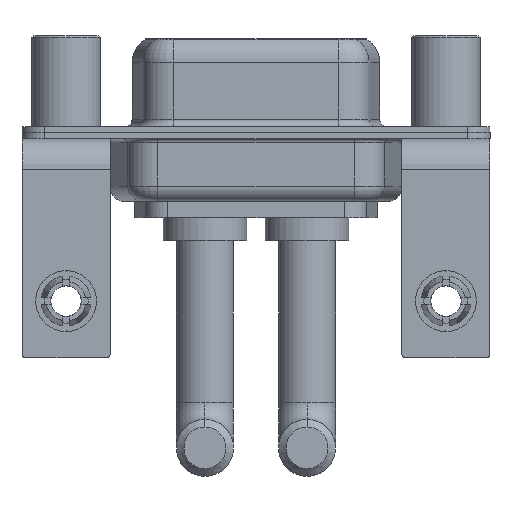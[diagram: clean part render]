
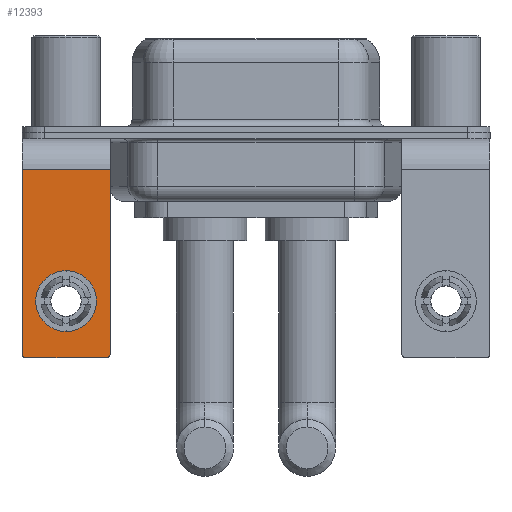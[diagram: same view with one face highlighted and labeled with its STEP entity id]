
A CAD part, front view. The second image highlights one B-rep face of the part: STEP entity #12393.
In plain terms, the highlighted planar face has unit normal (0, -1, 0).
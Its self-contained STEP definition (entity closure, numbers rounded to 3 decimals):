
#445 = CARTESIAN_POINT ( 'NONE',  ( 0., -6.25, -11.07 ) ) ;
#511 = CARTESIAN_POINT ( 'NONE',  ( 2.9, -6.25, -2.4 ) ) ;
#1584 = DIRECTION ( 'NONE',  ( 0., -1., 0. ) ) ;
#2166 = PLANE ( 'NONE',  #10290 ) ;
#2260 = DIRECTION ( 'NONE',  ( 0., 0., -1. ) ) ;
#2263 = CARTESIAN_POINT ( 'NONE',  ( 2.9, -6.25, -14.55 ) ) ;
#2295 = EDGE_CURVE ( 'NONE', #8307, #11907, #9735, .T. ) ;
#2417 = EDGE_LOOP ( 'NONE', ( #10380, #12524 ) ) ;
#2594 = AXIS2_PLACEMENT_3D ( 'NONE', #2831, #1584, #11796 ) ;
#2643 = DIRECTION ( 'NONE',  ( 0., 0., 1. ) ) ;
#2718 = CIRCLE ( 'NONE', #9557, 2. ) ;
#2831 = CARTESIAN_POINT ( 'NONE',  ( 2.65, -6.25, -14.55 ) ) ;
#3106 = DIRECTION ( 'NONE',  ( 0., 0., 1. ) ) ;
#3532 = ORIENTED_EDGE ( 'NONE', *, *, #2295, .F. ) ;
#3702 = LINE ( 'NONE', #4856, #12102 ) ;
#3968 = EDGE_CURVE ( 'NONE', #8307, #15414, #9694, .T. ) ;
#4039 = ORIENTED_EDGE ( 'NONE', *, *, #3968, .T. ) ;
#4410 = EDGE_LOOP ( 'NONE', ( #13294, #12450, #3532, #4039, #4470, #15979 ) ) ;
#4470 = ORIENTED_EDGE ( 'NONE', *, *, #13172, .F. ) ;
#4719 = FACE_BOUND ( 'NONE', #2417, .T. ) ;
#4856 = CARTESIAN_POINT ( 'NONE',  ( 2.9, -6.25, -2.4 ) ) ;
#4880 = DIRECTION ( 'NONE',  ( 0., 1., 0. ) ) ;
#4890 = CARTESIAN_POINT ( 'NONE',  ( -2.9, -6.25, -2.4 ) ) ;
#5168 = VERTEX_POINT ( 'NONE', #7751 ) ;
#5939 = FACE_OUTER_BOUND ( 'NONE', #4410, .T. ) ;
#6107 = CARTESIAN_POINT ( 'NONE',  ( 2.9, -6.25, -14.8 ) ) ;
#6533 = VECTOR ( 'NONE', #13696, 1000. ) ;
#6582 = CARTESIAN_POINT ( 'NONE',  ( 0., -6.25, -11.07 ) ) ;
#7569 = CARTESIAN_POINT ( 'NONE',  ( -2.65, -6.25, -14.55 ) ) ;
#7655 = EDGE_CURVE ( 'NONE', #11642, #9091, #12543, .T. ) ;
#7751 = CARTESIAN_POINT ( 'NONE',  ( 0., -6.25, -13.07 ) ) ;
#7813 = DIRECTION ( 'NONE',  ( 0., -1., 0. ) ) ;
#7855 = CARTESIAN_POINT ( 'NONE',  ( -2.65, -6.25, -14.8 ) ) ;
#7867 = CIRCLE ( 'NONE', #12327, 0.25 ) ;
#7914 = DIRECTION ( 'NONE',  ( 0., 1., 0. ) ) ;
#8307 = VERTEX_POINT ( 'NONE', #11599 ) ;
#9091 = VERTEX_POINT ( 'NONE', #13529 ) ;
#9424 = CARTESIAN_POINT ( 'NONE',  ( -2.9, -6.25, -2.4 ) ) ;
#9557 = AXIS2_PLACEMENT_3D ( 'NONE', #6582, #7914, #2643 ) ;
#9694 = CIRCLE ( 'NONE', #2594, 0.25 ) ;
#9735 = LINE ( 'NONE', #6107, #6533 ) ;
#9746 = EDGE_CURVE ( 'NONE', #9091, #11907, #7867, .T. ) ;
#9886 = EDGE_CURVE ( 'NONE', #5168, #13021, #15776, .T. ) ;
#10270 = CARTESIAN_POINT ( 'NONE',  ( 2.9, -6.25, -2.4 ) ) ;
#10290 = AXIS2_PLACEMENT_3D ( 'NONE', #12124, #4880, #10971 ) ;
#10380 = ORIENTED_EDGE ( 'NONE', *, *, #9886, .T. ) ;
#10957 = EDGE_CURVE ( 'NONE', #15113, #11642, #3702, .T. ) ;
#10971 = DIRECTION ( 'NONE',  ( 0., 0., 1. ) ) ;
#11599 = CARTESIAN_POINT ( 'NONE',  ( 2.65, -6.25, -14.8 ) ) ;
#11642 = VERTEX_POINT ( 'NONE', #9424 ) ;
#11796 = DIRECTION ( 'NONE',  ( 0., 0., 1. ) ) ;
#11907 = VERTEX_POINT ( 'NONE', #7855 ) ;
#12102 = VECTOR ( 'NONE', #16071, 1000. ) ;
#12124 = CARTESIAN_POINT ( 'NONE',  ( 2.9, -6.25, -2.4 ) ) ;
#12327 = AXIS2_PLACEMENT_3D ( 'NONE', #7569, #7813, #12817 ) ;
#12393 = ADVANCED_FACE ( 'NONE', ( #4719, #5939 ), #2166, .F. ) ;
#12450 = ORIENTED_EDGE ( 'NONE', *, *, #9746, .T. ) ;
#12524 = ORIENTED_EDGE ( 'NONE', *, *, #16166, .T. ) ;
#12543 = LINE ( 'NONE', #4890, #12966 ) ;
#12672 = DIRECTION ( 'NONE',  ( 0., 0., -1. ) ) ;
#12755 = LINE ( 'NONE', #10270, #15854 ) ;
#12817 = DIRECTION ( 'NONE',  ( 0., 0., 1. ) ) ;
#12966 = VECTOR ( 'NONE', #2260, 1000. ) ;
#13021 = VERTEX_POINT ( 'NONE', #14589 ) ;
#13172 = EDGE_CURVE ( 'NONE', #15113, #15414, #12755, .T. ) ;
#13294 = ORIENTED_EDGE ( 'NONE', *, *, #7655, .T. ) ;
#13529 = CARTESIAN_POINT ( 'NONE',  ( -2.9, -6.25, -14.55 ) ) ;
#13696 = DIRECTION ( 'NONE',  ( -1., 0., 0. ) ) ;
#14179 = AXIS2_PLACEMENT_3D ( 'NONE', #445, #15723, #3106 ) ;
#14589 = CARTESIAN_POINT ( 'NONE',  ( 0., -6.25, -9.07 ) ) ;
#15113 = VERTEX_POINT ( 'NONE', #511 ) ;
#15414 = VERTEX_POINT ( 'NONE', #2263 ) ;
#15723 = DIRECTION ( 'NONE',  ( 0., 1., 0. ) ) ;
#15776 = CIRCLE ( 'NONE', #14179, 2. ) ;
#15854 = VECTOR ( 'NONE', #12672, 1000. ) ;
#15979 = ORIENTED_EDGE ( 'NONE', *, *, #10957, .T. ) ;
#16071 = DIRECTION ( 'NONE',  ( -1., 0., 0. ) ) ;
#16166 = EDGE_CURVE ( 'NONE', #13021, #5168, #2718, .T. ) ;
